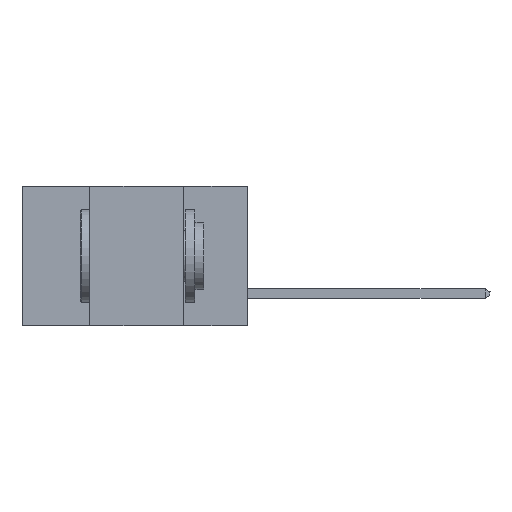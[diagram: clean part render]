
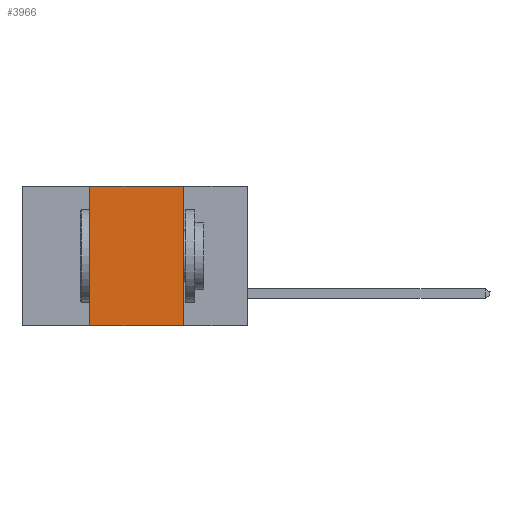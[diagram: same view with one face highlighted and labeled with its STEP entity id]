
A CAD part, left-side view. The second image highlights one B-rep face of the part: STEP entity #3966.
In plain terms, the highlighted planar face has unit normal (-1, 0, 0).
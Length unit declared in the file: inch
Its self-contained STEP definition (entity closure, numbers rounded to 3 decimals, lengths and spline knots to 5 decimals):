
#21 = ORIENTED_EDGE ( 'NONE', *, *, #4088, .T. ) ;
#1219 = LINE ( 'NONE', #7438, #9977 ) ;
#1602 = DIRECTION ( 'NONE',  ( 0., 0., -1. ) ) ;
#1973 = VERTEX_POINT ( 'NONE', #18725 ) ;
#3655 = ORIENTED_EDGE ( 'NONE', *, *, #7858, .F. ) ;
#3966 = ADVANCED_FACE ( 'NONE', ( #12180 ), #14474, .F. ) ;
#4088 = EDGE_CURVE ( 'NONE', #21398, #6985, #4821, .T. ) ;
#4821 = LINE ( 'NONE', #9654, #19182 ) ;
#5376 = EDGE_CURVE ( 'NONE', #21398, #13676, #1219, .T. ) ;
#6592 = EDGE_CURVE ( 'NONE', #13676, #1973, #12070, .T. ) ;
#6931 = CARTESIAN_POINT ( 'NONE',  ( 0., 0.42, 0. ) ) ;
#6985 = VERTEX_POINT ( 'NONE', #17926 ) ;
#7055 = DIRECTION ( 'NONE',  ( 0., 0., 1. ) ) ;
#7188 = CARTESIAN_POINT ( 'NONE',  ( 0., 0.17, -0.37 ) ) ;
#7438 = CARTESIAN_POINT ( 'NONE',  ( 0., 0.42, -0.37 ) ) ;
#7858 = EDGE_CURVE ( 'NONE', #1973, #6985, #13773, .T. ) ;
#8155 = VECTOR ( 'NONE', #1602, 39.37008 ) ;
#9266 = DIRECTION ( 'NONE',  ( 0., -1., 0. ) ) ;
#9654 = CARTESIAN_POINT ( 'NONE',  ( 0., 0.6, -0.37 ) ) ;
#9807 = DIRECTION ( 'NONE',  ( 0., -1., 0. ) ) ;
#9977 = VECTOR ( 'NONE', #7055, 39.37008 ) ;
#10427 = AXIS2_PLACEMENT_3D ( 'NONE', #15741, #13949, #13898 ) ;
#12070 = LINE ( 'NONE', #24043, #16489 ) ;
#12180 = FACE_OUTER_BOUND ( 'NONE', #14995, .T. ) ;
#13570 = CARTESIAN_POINT ( 'NONE',  ( 0., 0.42, -0.37 ) ) ;
#13676 = VERTEX_POINT ( 'NONE', #6931 ) ;
#13773 = LINE ( 'NONE', #7188, #8155 ) ;
#13898 = DIRECTION ( 'NONE',  ( 0., 0., -1. ) ) ;
#13949 = DIRECTION ( 'NONE',  ( 1., 0., 0. ) ) ;
#14474 = PLANE ( 'NONE',  #10427 ) ;
#14995 = EDGE_LOOP ( 'NONE', ( #3655, #18085, #19988, #21 ) ) ;
#15741 = CARTESIAN_POINT ( 'NONE',  ( 0., 0.6, 0. ) ) ;
#16489 = VECTOR ( 'NONE', #9266, 39.37008 ) ;
#17926 = CARTESIAN_POINT ( 'NONE',  ( 0., 0.17, -0.37 ) ) ;
#18085 = ORIENTED_EDGE ( 'NONE', *, *, #6592, .F. ) ;
#18725 = CARTESIAN_POINT ( 'NONE',  ( 0., 0.17, 0. ) ) ;
#19182 = VECTOR ( 'NONE', #9807, 39.37008 ) ;
#19988 = ORIENTED_EDGE ( 'NONE', *, *, #5376, .F. ) ;
#21398 = VERTEX_POINT ( 'NONE', #13570 ) ;
#24043 = CARTESIAN_POINT ( 'NONE',  ( 0., 0.6, 0. ) ) ;
